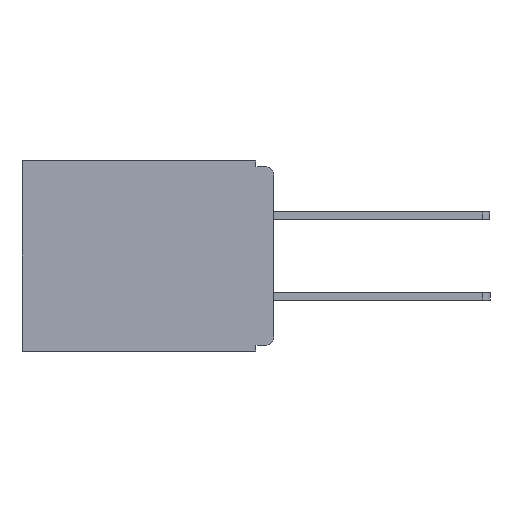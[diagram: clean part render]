
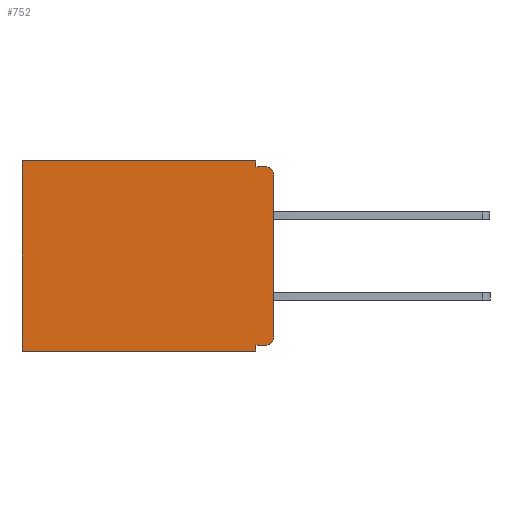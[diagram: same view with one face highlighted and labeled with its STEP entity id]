
A CAD part, left-side view. The second image highlights one B-rep face of the part: STEP entity #752.
In plain terms, the highlighted planar face has unit normal (-1, 0, 0).
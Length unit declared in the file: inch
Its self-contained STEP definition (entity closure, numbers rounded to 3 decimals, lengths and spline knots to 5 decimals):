
#137 = LINE ( 'NONE', #1591, #3759 ) ;
#138 = DIRECTION ( 'NONE',  ( 0., 0., -1. ) ) ;
#428 = CARTESIAN_POINT ( 'NONE',  ( 0.3, 0.015, -0.305 ) ) ;
#752 = ADVANCED_FACE ( 'NONE', ( #10148 ), #1291, .F. ) ;
#958 = CARTESIAN_POINT ( 'NONE',  ( 0.3, 0., -0.33 ) ) ;
#1291 = PLANE ( 'NONE',  #2457 ) ;
#1336 = VECTOR ( 'NONE', #138, 39.37008 ) ;
#1545 = AXIS2_PLACEMENT_3D ( 'NONE', #428, #7029, #13381 ) ;
#1591 = CARTESIAN_POINT ( 'NONE',  ( 0.3, 0., -0.01 ) ) ;
#1661 = VERTEX_POINT ( 'NONE', #10128 ) ;
#1751 = CARTESIAN_POINT ( 'NONE',  ( 0.3, 0., 0. ) ) ;
#1790 = DIRECTION ( 'NONE',  ( 0., 1., 0. ) ) ;
#1965 = LINE ( 'NONE', #958, #8773 ) ;
#2048 = CARTESIAN_POINT ( 'NONE',  ( 0.3, 0.031, 0. ) ) ;
#2358 = LINE ( 'NONE', #8209, #9547 ) ;
#2457 = AXIS2_PLACEMENT_3D ( 'NONE', #3975, #8417, #16706 ) ;
#2711 = DIRECTION ( 'NONE',  ( 0., 0., -1. ) ) ;
#2800 = LINE ( 'NONE', #9614, #9949 ) ;
#3517 = VERTEX_POINT ( 'NONE', #4171 ) ;
#3759 = VECTOR ( 'NONE', #14380, 39.37008 ) ;
#3778 = VERTEX_POINT ( 'NONE', #8434 ) ;
#3975 = CARTESIAN_POINT ( 'NONE',  ( 0.3, 0., -0.33 ) ) ;
#3985 = VERTEX_POINT ( 'NONE', #16454 ) ;
#4171 = CARTESIAN_POINT ( 'NONE',  ( 0.3, 0.031, -0.01 ) ) ;
#4290 = ORIENTED_EDGE ( 'NONE', *, *, #5362, .F. ) ;
#4377 = CARTESIAN_POINT ( 'NONE',  ( 0.3, 0.031, 0. ) ) ;
#4490 = CARTESIAN_POINT ( 'NONE',  ( 0.3, 0.031, -0.32 ) ) ;
#4723 = ORIENTED_EDGE ( 'NONE', *, *, #12862, .F. ) ;
#4847 = VECTOR ( 'NONE', #17726, 39.37008 ) ;
#5013 = EDGE_CURVE ( 'NONE', #3985, #15852, #11543, .T. ) ;
#5247 = EDGE_CURVE ( 'NONE', #17627, #17002, #15348, .T. ) ;
#5362 = EDGE_CURVE ( 'NONE', #16525, #7902, #2358, .T. ) ;
#5659 = ORIENTED_EDGE ( 'NONE', *, *, #6265, .T. ) ;
#5721 = CARTESIAN_POINT ( 'NONE',  ( 0.3, 0.015, -0.32 ) ) ;
#6265 = EDGE_CURVE ( 'NONE', #12904, #3985, #11731, .T. ) ;
#6296 = EDGE_CURVE ( 'NONE', #12904, #3517, #12789, .T. ) ;
#7029 = DIRECTION ( 'NONE',  ( -1., 0., 0. ) ) ;
#7081 = DIRECTION ( 'NONE',  ( 0., 0., -1. ) ) ;
#7208 = CARTESIAN_POINT ( 'NONE',  ( 0.3, 0.437, -0.33 ) ) ;
#7226 = EDGE_LOOP ( 'NONE', ( #10241, #17027, #13493, #13068, #5659, #15774, #4723, #4290, #15989, #12434 ) ) ;
#7362 = VECTOR ( 'NONE', #7081, 39.37008 ) ;
#7870 = EDGE_CURVE ( 'NONE', #3778, #17002, #12322, .T. ) ;
#7902 = VERTEX_POINT ( 'NONE', #17539 ) ;
#8087 = EDGE_CURVE ( 'NONE', #3778, #1661, #12964, .T. ) ;
#8209 = CARTESIAN_POINT ( 'NONE',  ( 0.3, 0.031, -0.33 ) ) ;
#8417 = DIRECTION ( 'NONE',  ( 1., 0., 0. ) ) ;
#8434 = CARTESIAN_POINT ( 'NONE',  ( 0.3, 0., -0.025 ) ) ;
#8773 = VECTOR ( 'NONE', #12484, 39.37008 ) ;
#9547 = VECTOR ( 'NONE', #2711, 39.37008 ) ;
#9614 = CARTESIAN_POINT ( 'NONE',  ( 0.3, 0., -0.32 ) ) ;
#9904 = CARTESIAN_POINT ( 'NONE',  ( 0.3, 0., -0.305 ) ) ;
#9949 = VECTOR ( 'NONE', #11087, 39.37008 ) ;
#10128 = CARTESIAN_POINT ( 'NONE',  ( 0.3, 0.015, -0.01 ) ) ;
#10148 = FACE_OUTER_BOUND ( 'NONE', #7226, .T. ) ;
#10241 = ORIENTED_EDGE ( 'NONE', *, *, #7870, .F. ) ;
#10886 = EDGE_CURVE ( 'NONE', #17627, #16525, #2800, .T. ) ;
#11087 = DIRECTION ( 'NONE',  ( 0., 1., 0. ) ) ;
#11543 = LINE ( 'NONE', #7208, #7362 ) ;
#11731 = LINE ( 'NONE', #1751, #17160 ) ;
#12322 = LINE ( 'NONE', #17597, #4847 ) ;
#12434 = ORIENTED_EDGE ( 'NONE', *, *, #5247, .T. ) ;
#12484 = DIRECTION ( 'NONE',  ( 0., 1., 0. ) ) ;
#12567 = CARTESIAN_POINT ( 'NONE',  ( 0.3, 0.437, -0.33 ) ) ;
#12742 = AXIS2_PLACEMENT_3D ( 'NONE', #15883, #15867, #15842 ) ;
#12789 = LINE ( 'NONE', #2048, #1336 ) ;
#12862 = EDGE_CURVE ( 'NONE', #7902, #15852, #1965, .T. ) ;
#12904 = VERTEX_POINT ( 'NONE', #4377 ) ;
#12964 = CIRCLE ( 'NONE', #12742, 0.015 ) ;
#13068 = ORIENTED_EDGE ( 'NONE', *, *, #6296, .F. ) ;
#13381 = DIRECTION ( 'NONE',  ( 0., 0., -1. ) ) ;
#13493 = ORIENTED_EDGE ( 'NONE', *, *, #17791, .F. ) ;
#14380 = DIRECTION ( 'NONE',  ( 0., -1., 0. ) ) ;
#15348 = CIRCLE ( 'NONE', #1545, 0.015 ) ;
#15774 = ORIENTED_EDGE ( 'NONE', *, *, #5013, .T. ) ;
#15842 = DIRECTION ( 'NONE',  ( 0., 0., -1. ) ) ;
#15852 = VERTEX_POINT ( 'NONE', #12567 ) ;
#15867 = DIRECTION ( 'NONE',  ( -1., 0., 0. ) ) ;
#15883 = CARTESIAN_POINT ( 'NONE',  ( 0.3, 0.015, -0.025 ) ) ;
#15989 = ORIENTED_EDGE ( 'NONE', *, *, #10886, .F. ) ;
#16454 = CARTESIAN_POINT ( 'NONE',  ( 0.3, 0.437, 0. ) ) ;
#16525 = VERTEX_POINT ( 'NONE', #4490 ) ;
#16706 = DIRECTION ( 'NONE',  ( 0., 0., -1. ) ) ;
#17002 = VERTEX_POINT ( 'NONE', #9904 ) ;
#17027 = ORIENTED_EDGE ( 'NONE', *, *, #8087, .T. ) ;
#17160 = VECTOR ( 'NONE', #1790, 39.37008 ) ;
#17539 = CARTESIAN_POINT ( 'NONE',  ( 0.3, 0.031, -0.33 ) ) ;
#17597 = CARTESIAN_POINT ( 'NONE',  ( 0.3, 0., -0.33 ) ) ;
#17627 = VERTEX_POINT ( 'NONE', #5721 ) ;
#17726 = DIRECTION ( 'NONE',  ( 0., 0., -1. ) ) ;
#17791 = EDGE_CURVE ( 'NONE', #3517, #1661, #137, .T. ) ;
